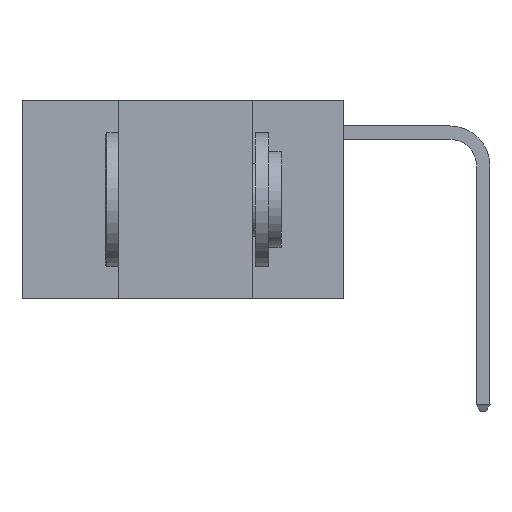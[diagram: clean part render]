
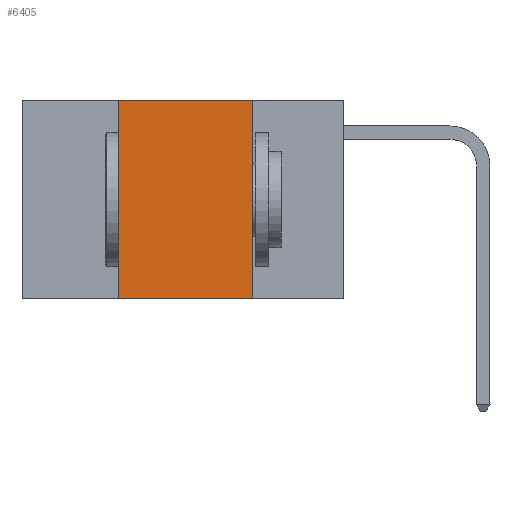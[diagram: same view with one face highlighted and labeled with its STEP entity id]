
A CAD part, left-side view. The second image highlights one B-rep face of the part: STEP entity #6405.
In plain terms, the highlighted planar face has unit normal (-1, 0, 0).
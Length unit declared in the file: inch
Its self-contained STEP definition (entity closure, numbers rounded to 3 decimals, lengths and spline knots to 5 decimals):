
#1563 = DIRECTION ( 'NONE',  ( 1., 0., 0. ) ) ;
#1675 = EDGE_CURVE ( 'NONE', #3797, #15065, #3174, .T. ) ;
#1861 = LINE ( 'NONE', #13243, #15884 ) ;
#2079 = CARTESIAN_POINT ( 'NONE',  ( 0., 0.17, 0. ) ) ;
#2158 = CARTESIAN_POINT ( 'NONE',  ( 0., 0.6, 0. ) ) ;
#2620 = CARTESIAN_POINT ( 'NONE',  ( 0., 0.6, -0.37 ) ) ;
#2664 = PLANE ( 'NONE',  #11958 ) ;
#2707 = EDGE_CURVE ( 'NONE', #7474, #12941, #8994, .T. ) ;
#3174 = LINE ( 'NONE', #2158, #7144 ) ;
#3283 = CARTESIAN_POINT ( 'NONE',  ( 0., 0.42, -0.37 ) ) ;
#3797 = VERTEX_POINT ( 'NONE', #9430 ) ;
#3798 = EDGE_CURVE ( 'NONE', #15065, #12941, #1861, .T. ) ;
#5531 = VECTOR ( 'NONE', #7674, 39.37008 ) ;
#5558 = DIRECTION ( 'NONE',  ( 0., 0., -1. ) ) ;
#5679 = EDGE_LOOP ( 'NONE', ( #13132, #8990, #7717, #13443 ) ) ;
#6018 = DIRECTION ( 'NONE',  ( 0., -1., 0. ) ) ;
#6405 = ADVANCED_FACE ( 'NONE', ( #6539 ), #2664, .F. ) ;
#6539 = FACE_OUTER_BOUND ( 'NONE', #5679, .T. ) ;
#7144 = VECTOR ( 'NONE', #6018, 39.37008 ) ;
#7474 = VERTEX_POINT ( 'NONE', #3283 ) ;
#7506 = CARTESIAN_POINT ( 'NONE',  ( 0., 0.17, -0.37 ) ) ;
#7674 = DIRECTION ( 'NONE',  ( 0., -1., 0. ) ) ;
#7717 = ORIENTED_EDGE ( 'NONE', *, *, #8579, .F. ) ;
#7947 = VECTOR ( 'NONE', #16318, 39.37008 ) ;
#8579 = EDGE_CURVE ( 'NONE', #7474, #3797, #11140, .T. ) ;
#8990 = ORIENTED_EDGE ( 'NONE', *, *, #1675, .F. ) ;
#8994 = LINE ( 'NONE', #2620, #5531 ) ;
#9430 = CARTESIAN_POINT ( 'NONE',  ( 0., 0.42, 0. ) ) ;
#11140 = LINE ( 'NONE', #12598, #7947 ) ;
#11958 = AXIS2_PLACEMENT_3D ( 'NONE', #15634, #1563, #13184 ) ;
#12598 = CARTESIAN_POINT ( 'NONE',  ( 0., 0.42, 0. ) ) ;
#12941 = VERTEX_POINT ( 'NONE', #7506 ) ;
#13132 = ORIENTED_EDGE ( 'NONE', *, *, #3798, .F. ) ;
#13184 = DIRECTION ( 'NONE',  ( 0., 0., -1. ) ) ;
#13243 = CARTESIAN_POINT ( 'NONE',  ( 0., 0.17, 0. ) ) ;
#13443 = ORIENTED_EDGE ( 'NONE', *, *, #2707, .T. ) ;
#15065 = VERTEX_POINT ( 'NONE', #2079 ) ;
#15634 = CARTESIAN_POINT ( 'NONE',  ( 0., 0.6, 0. ) ) ;
#15884 = VECTOR ( 'NONE', #5558, 39.37008 ) ;
#16318 = DIRECTION ( 'NONE',  ( 0., 0., 1. ) ) ;
